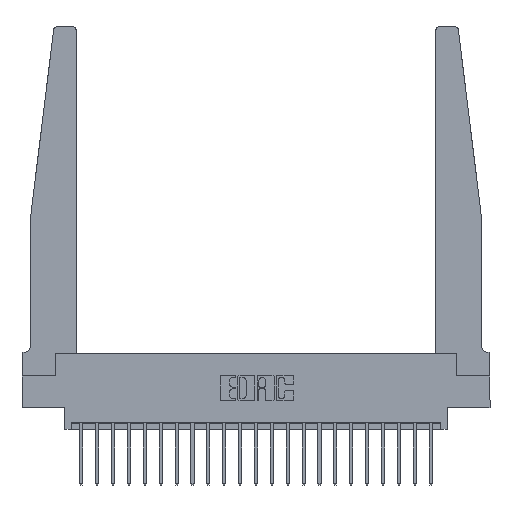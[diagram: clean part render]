
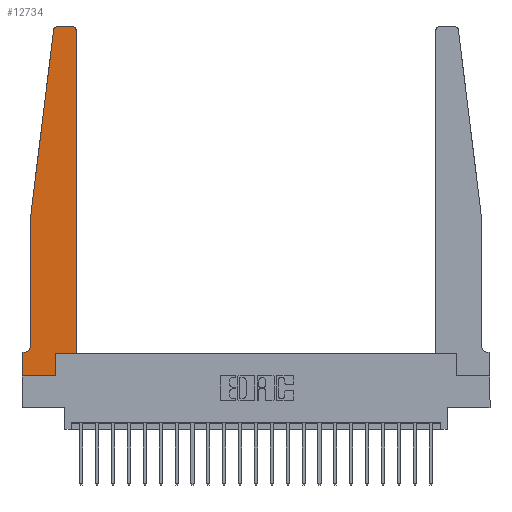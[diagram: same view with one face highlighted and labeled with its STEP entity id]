
A CAD part, top view. The second image highlights one B-rep face of the part: STEP entity #12734.
In plain terms, the highlighted planar face has unit normal (0, 0, 1).
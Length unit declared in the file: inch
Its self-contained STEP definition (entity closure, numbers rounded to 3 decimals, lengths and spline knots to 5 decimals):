
#530 = LINE ( 'NONE', #2497, #8322 ) ;
#612 = AXIS2_PLACEMENT_3D ( 'NONE', #5051, #10501, #5276 ) ;
#805 = DIRECTION ( 'NONE',  ( 0., 0., 1. ) ) ;
#1210 = DIRECTION ( 'NONE',  ( 0., -1., 0. ) ) ;
#2031 = DIRECTION ( 'NONE',  ( -1., 0., 0. ) ) ;
#2459 = ORIENTED_EDGE ( 'NONE', *, *, #11812, .T. ) ;
#2487 = CARTESIAN_POINT ( 'NONE',  ( 0., 0., 0.37 ) ) ;
#2497 = CARTESIAN_POINT ( 'NONE',  ( 0.25, 2.75, 0.37 ) ) ;
#2562 = VERTEX_POINT ( 'NONE', #2787 ) ;
#2661 = CARTESIAN_POINT ( 'NONE',  ( 0.27653, 2.72, 0.37 ) ) ;
#2705 = CARTESIAN_POINT ( 'NONE',  ( 0.425, 0.18, 0.37 ) ) ;
#2720 = LINE ( 'NONE', #15022, #5197 ) ;
#2787 = CARTESIAN_POINT ( 'NONE',  ( 0.2605, 0.18, 0.37 ) ) ;
#2850 = EDGE_CURVE ( 'NONE', #13215, #8625, #11425, .T. ) ;
#2920 = LINE ( 'NONE', #13242, #21924 ) ;
#2930 = LINE ( 'NONE', #9779, #21332 ) ;
#3038 = LINE ( 'NONE', #21127, #12962 ) ;
#3267 = CARTESIAN_POINT ( 'NONE',  ( 0.065, 0.2375, 0.37 ) ) ;
#3404 = VECTOR ( 'NONE', #20108, 39.37008 ) ;
#3476 = DIRECTION ( 'NONE',  ( 0., 0., 1. ) ) ;
#4321 = ORIENTED_EDGE ( 'NONE', *, *, #2850, .T. ) ;
#4761 = CARTESIAN_POINT ( 'NONE',  ( 0.24675, 2.72367, 0.37 ) ) ;
#4766 = ORIENTED_EDGE ( 'NONE', *, *, #22324, .T. ) ;
#5051 = CARTESIAN_POINT ( 'NONE',  ( 0., 0.1875, 0.37 ) ) ;
#5197 = VECTOR ( 'NONE', #1210, 39.37008 ) ;
#5233 = DIRECTION ( 'NONE',  ( 1., 0., 0. ) ) ;
#5276 = DIRECTION ( 'NONE',  ( 1., 0., 0. ) ) ;
#6066 = VERTEX_POINT ( 'NONE', #2487 ) ;
#6170 = VERTEX_POINT ( 'NONE', #22670 ) ;
#6393 = DIRECTION ( 'NONE',  ( -0.122, -0.992, 0. ) ) ;
#6403 = EDGE_CURVE ( 'NONE', #9995, #11954, #2920, .T. ) ;
#6445 = CIRCLE ( 'NONE', #22019, 0.05 ) ;
#6465 = EDGE_CURVE ( 'NONE', #10467, #9995, #15218, .T. ) ;
#6802 = EDGE_CURVE ( 'NONE', #12504, #10467, #19318, .T. ) ;
#6903 = FACE_OUTER_BOUND ( 'NONE', #18365, .T. ) ;
#6925 = ORIENTED_EDGE ( 'NONE', *, *, #6403, .T. ) ;
#6979 = CARTESIAN_POINT ( 'NONE',  ( 0.2605, 0.18, 0.37 ) ) ;
#7359 = PLANE ( 'NONE',  #612 ) ;
#7497 = VECTOR ( 'NONE', #8708, 39.37008 ) ;
#8070 = CARTESIAN_POINT ( 'NONE',  ( 0.065, 1.25, 0.37 ) ) ;
#8075 = ORIENTED_EDGE ( 'NONE', *, *, #9903, .T. ) ;
#8162 = ORIENTED_EDGE ( 'NONE', *, *, #16962, .T. ) ;
#8322 = VECTOR ( 'NONE', #2031, 39.37008 ) ;
#8535 = CARTESIAN_POINT ( 'NONE',  ( 0.27653, 2.75, 0.37 ) ) ;
#8582 = VECTOR ( 'NONE', #6393, 39.37008 ) ;
#8625 = VERTEX_POINT ( 'NONE', #17361 ) ;
#8708 = DIRECTION ( 'NONE',  ( 1., 0., 0. ) ) ;
#8883 = CARTESIAN_POINT ( 'NONE',  ( 0.015, 0.1875, 0.37 ) ) ;
#9272 = ORIENTED_EDGE ( 'NONE', *, *, #17803, .T. ) ;
#9558 = CARTESIAN_POINT ( 'NONE',  ( 0., 0.1875, 0.37 ) ) ;
#9779 = CARTESIAN_POINT ( 'NONE',  ( 0.065, 0.1875, 0.37 ) ) ;
#9903 = EDGE_CURVE ( 'NONE', #8625, #12504, #530, .T. ) ;
#9995 = VERTEX_POINT ( 'NONE', #8070 ) ;
#10032 = EDGE_CURVE ( 'NONE', #11954, #12659, #6445, .T. ) ;
#10195 = EDGE_CURVE ( 'NONE', #6170, #2562, #14293, .T. ) ;
#10351 = DIRECTION ( 'NONE',  ( -1., 0., 0. ) ) ;
#10467 = VERTEX_POINT ( 'NONE', #4761 ) ;
#10501 = DIRECTION ( 'NONE',  ( 0., 0., 1. ) ) ;
#10558 = DIRECTION ( 'NONE',  ( 1., 0., 0. ) ) ;
#10560 = LINE ( 'NONE', #22752, #7497 ) ;
#11367 = DIRECTION ( 'NONE',  ( 1., 0., 0. ) ) ;
#11425 = CIRCLE ( 'NONE', #20699, 0.03 ) ;
#11812 = EDGE_CURVE ( 'NONE', #12659, #21583, #2930, .T. ) ;
#11954 = VERTEX_POINT ( 'NONE', #3267 ) ;
#12504 = VERTEX_POINT ( 'NONE', #8535 ) ;
#12659 = VERTEX_POINT ( 'NONE', #8883 ) ;
#12734 = ADVANCED_FACE ( 'NONE', ( #6903 ), #7359, .T. ) ;
#12905 = ORIENTED_EDGE ( 'NONE', *, *, #10032, .T. ) ;
#12962 = VECTOR ( 'NONE', #5233, 39.37008 ) ;
#13215 = VERTEX_POINT ( 'NONE', #14649 ) ;
#13242 = CARTESIAN_POINT ( 'NONE',  ( 0.065, 1.25, 0.37 ) ) ;
#13363 = DIRECTION ( 'NONE',  ( 0., -1., 0. ) ) ;
#13929 = VECTOR ( 'NONE', #21368, 39.37008 ) ;
#14293 = LINE ( 'NONE', #6979, #13929 ) ;
#14649 = CARTESIAN_POINT ( 'NONE',  ( 0.425, 2.72, 0.37 ) ) ;
#15022 = CARTESIAN_POINT ( 'NONE',  ( 0., 0., 0.37 ) ) ;
#15071 = VERTEX_POINT ( 'NONE', #16527 ) ;
#15218 = LINE ( 'NONE', #22300, #8582 ) ;
#15687 = CARTESIAN_POINT ( 'NONE',  ( 0.015, 0.2375, 0.37 ) ) ;
#15736 = ORIENTED_EDGE ( 'NONE', *, *, #10195, .T. ) ;
#16527 = CARTESIAN_POINT ( 'NONE',  ( 0.425, 0.18, 0.37 ) ) ;
#16962 = EDGE_CURVE ( 'NONE', #6066, #6170, #3038, .T. ) ;
#17086 = DIRECTION ( 'NONE',  ( -1., 0., 0. ) ) ;
#17361 = CARTESIAN_POINT ( 'NONE',  ( 0.395, 2.75, 0.37 ) ) ;
#17803 = EDGE_CURVE ( 'NONE', #21583, #6066, #2720, .T. ) ;
#18027 = ORIENTED_EDGE ( 'NONE', *, *, #21602, .T. ) ;
#18212 = AXIS2_PLACEMENT_3D ( 'NONE', #2661, #805, #11367 ) ;
#18365 = EDGE_LOOP ( 'NONE', ( #8075, #22549, #19514, #6925, #12905, #2459, #9272, #8162, #15736, #4766, #18027, #4321 ) ) ;
#19158 = DIRECTION ( 'NONE',  ( 0., 0., -1. ) ) ;
#19318 = CIRCLE ( 'NONE', #18212, 0.03 ) ;
#19373 = CARTESIAN_POINT ( 'NONE',  ( 0.395, 2.72, 0.37 ) ) ;
#19514 = ORIENTED_EDGE ( 'NONE', *, *, #6465, .T. ) ;
#20108 = DIRECTION ( 'NONE',  ( 0., 1., 0. ) ) ;
#20340 = LINE ( 'NONE', #2705, #3404 ) ;
#20699 = AXIS2_PLACEMENT_3D ( 'NONE', #19373, #3476, #10558 ) ;
#21127 = CARTESIAN_POINT ( 'NONE',  ( 0., 0., 0.37 ) ) ;
#21332 = VECTOR ( 'NONE', #17086, 39.37008 ) ;
#21368 = DIRECTION ( 'NONE',  ( 0., 1., 0. ) ) ;
#21583 = VERTEX_POINT ( 'NONE', #9558 ) ;
#21602 = EDGE_CURVE ( 'NONE', #15071, #13215, #20340, .T. ) ;
#21924 = VECTOR ( 'NONE', #13363, 39.37008 ) ;
#22019 = AXIS2_PLACEMENT_3D ( 'NONE', #15687, #19158, #10351 ) ;
#22300 = CARTESIAN_POINT ( 'NONE',  ( 0.065, 1.25, 0.37 ) ) ;
#22324 = EDGE_CURVE ( 'NONE', #2562, #15071, #10560, .T. ) ;
#22549 = ORIENTED_EDGE ( 'NONE', *, *, #6802, .T. ) ;
#22670 = CARTESIAN_POINT ( 'NONE',  ( 0.2605, 0., 0.37 ) ) ;
#22752 = CARTESIAN_POINT ( 'NONE',  ( 0.425, 0.18, 0.37 ) ) ;
